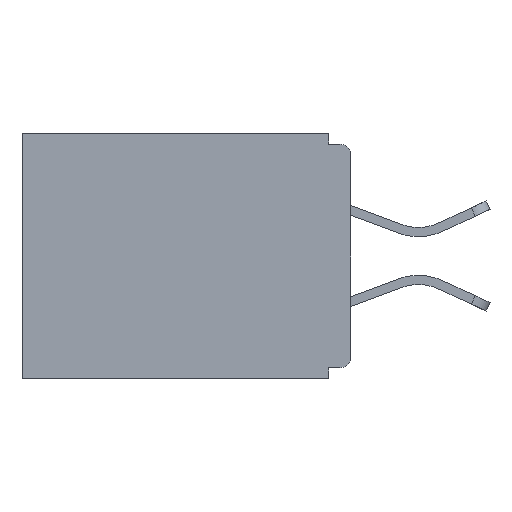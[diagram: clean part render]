
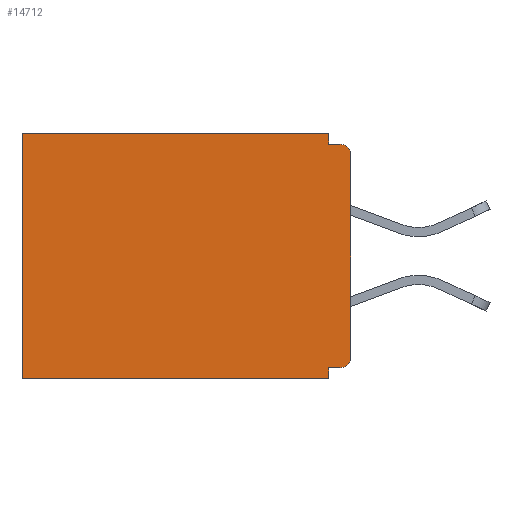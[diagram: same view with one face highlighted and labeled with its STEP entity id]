
A CAD part, left-side view. The second image highlights one B-rep face of the part: STEP entity #14712.
In plain terms, the highlighted planar face has unit normal (-1, 0, 0).
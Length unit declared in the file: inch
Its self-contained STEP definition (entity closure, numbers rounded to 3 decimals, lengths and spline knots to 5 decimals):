
#4 = CARTESIAN_POINT ( 'NONE',  ( 0.298, 0.031, -0.328 ) ) ;
#178 = LINE ( 'NONE', #515, #5808 ) ;
#179 = ORIENTED_EDGE ( 'NONE', *, *, #16428, .F. ) ;
#185 = CARTESIAN_POINT ( 'NONE',  ( 0.298, 0.031, -0.343 ) ) ;
#515 = CARTESIAN_POINT ( 'NONE',  ( 0.298, 0., -0.328 ) ) ;
#634 = CARTESIAN_POINT ( 'NONE',  ( 0.298, 0.46, 0. ) ) ;
#1150 = EDGE_CURVE ( 'NONE', #5513, #9753, #13021, .T. ) ;
#1374 = CARTESIAN_POINT ( 'NONE',  ( 0.298, 0.031, -0.343 ) ) ;
#1407 = EDGE_LOOP ( 'NONE', ( #13630, #1444, #7308, #13291, #6910, #11498, #1440, #179, #6808, #5266 ) ) ;
#1440 = ORIENTED_EDGE ( 'NONE', *, *, #1645, .F. ) ;
#1444 = ORIENTED_EDGE ( 'NONE', *, *, #9063, .F. ) ;
#1598 = VECTOR ( 'NONE', #7910, 39.37008 ) ;
#1629 = EDGE_CURVE ( 'NONE', #8692, #10953, #5450, .T. ) ;
#1645 = EDGE_CURVE ( 'NONE', #11223, #8692, #11439, .T. ) ;
#1943 = VECTOR ( 'NONE', #14411, 39.37008 ) ;
#2340 = VECTOR ( 'NONE', #9691, 39.37008 ) ;
#2417 = DIRECTION ( 'NONE',  ( 0., 0., -1. ) ) ;
#3238 = CARTESIAN_POINT ( 'NONE',  ( 0.298, 0., 0. ) ) ;
#3262 = EDGE_CURVE ( 'NONE', #7286, #14061, #7306, .T. ) ;
#3324 = VECTOR ( 'NONE', #3761, 39.37008 ) ;
#3612 = DIRECTION ( 'NONE',  ( -1., 0., 0. ) ) ;
#3679 = VECTOR ( 'NONE', #2417, 39.37008 ) ;
#3761 = DIRECTION ( 'NONE',  ( 0., 1., 0. ) ) ;
#4390 = LINE ( 'NONE', #634, #12402 ) ;
#4412 = PLANE ( 'NONE',  #11526 ) ;
#4455 = DIRECTION ( 'NONE',  ( 0., 1., 0. ) ) ;
#4909 = VERTEX_POINT ( 'NONE', #7822 ) ;
#5168 = CARTESIAN_POINT ( 'NONE',  ( 0.298, 0.015, -0.328 ) ) ;
#5172 = AXIS2_PLACEMENT_3D ( 'NONE', #9846, #3612, #14905 ) ;
#5266 = ORIENTED_EDGE ( 'NONE', *, *, #6485, .F. ) ;
#5450 = LINE ( 'NONE', #10848, #8223 ) ;
#5513 = VERTEX_POINT ( 'NONE', #13743 ) ;
#5716 = CARTESIAN_POINT ( 'NONE',  ( 0.298, 0., 0. ) ) ;
#5808 = VECTOR ( 'NONE', #8428, 39.37008 ) ;
#6282 = CARTESIAN_POINT ( 'NONE',  ( 0.298, 0., 0. ) ) ;
#6297 = CARTESIAN_POINT ( 'NONE',  ( 0.298, 0.031, -0.015 ) ) ;
#6485 = EDGE_CURVE ( 'NONE', #5513, #10709, #15809, .T. ) ;
#6808 = ORIENTED_EDGE ( 'NONE', *, *, #13981, .T. ) ;
#6819 = DIRECTION ( 'NONE',  ( 0., 0., -1. ) ) ;
#6910 = ORIENTED_EDGE ( 'NONE', *, *, #16467, .T. ) ;
#7286 = VERTEX_POINT ( 'NONE', #9744 ) ;
#7306 = LINE ( 'NONE', #1374, #3679 ) ;
#7308 = ORIENTED_EDGE ( 'NONE', *, *, #3262, .F. ) ;
#7575 = AXIS2_PLACEMENT_3D ( 'NONE', #11756, #14497, #6819 ) ;
#7822 = CARTESIAN_POINT ( 'NONE',  ( 0.298, 0.46, 0. ) ) ;
#7910 = DIRECTION ( 'NONE',  ( 0., 0., -1. ) ) ;
#7918 = CARTESIAN_POINT ( 'NONE',  ( 0.298, 0., -0.015 ) ) ;
#8223 = VECTOR ( 'NONE', #4455, 39.37008 ) ;
#8428 = DIRECTION ( 'NONE',  ( 0., 1., 0. ) ) ;
#8692 = VERTEX_POINT ( 'NONE', #13845 ) ;
#9063 = EDGE_CURVE ( 'NONE', #14061, #9753, #14378, .T. ) ;
#9455 = EDGE_CURVE ( 'NONE', #7286, #4909, #14975, .T. ) ;
#9556 = DIRECTION ( 'NONE',  ( 0., 0., -1. ) ) ;
#9691 = DIRECTION ( 'NONE',  ( 0., 0., -1. ) ) ;
#9744 = CARTESIAN_POINT ( 'NONE',  ( 0.298, 0.031, 0. ) ) ;
#9753 = VERTEX_POINT ( 'NONE', #12408 ) ;
#9846 = CARTESIAN_POINT ( 'NONE',  ( 0.298, 0.015, -0.313 ) ) ;
#9995 = CARTESIAN_POINT ( 'NONE',  ( 0.298, 0.46, -0.343 ) ) ;
#10709 = VERTEX_POINT ( 'NONE', #14428 ) ;
#10848 = CARTESIAN_POINT ( 'NONE',  ( 0.298, 0., -0.343 ) ) ;
#10953 = VERTEX_POINT ( 'NONE', #9995 ) ;
#11223 = VERTEX_POINT ( 'NONE', #4 ) ;
#11439 = LINE ( 'NONE', #185, #1598 ) ;
#11498 = ORIENTED_EDGE ( 'NONE', *, *, #1629, .F. ) ;
#11526 = AXIS2_PLACEMENT_3D ( 'NONE', #5716, #16015, #9556 ) ;
#11756 = CARTESIAN_POINT ( 'NONE',  ( 0.298, 0.015, -0.03 ) ) ;
#12219 = DIRECTION ( 'NONE',  ( 0., 0., -1. ) ) ;
#12402 = VECTOR ( 'NONE', #12219, 39.37008 ) ;
#12408 = CARTESIAN_POINT ( 'NONE',  ( 0.298, 0.015, -0.015 ) ) ;
#13021 = CIRCLE ( 'NONE', #7575, 0.015 ) ;
#13207 = CIRCLE ( 'NONE', #5172, 0.015 ) ;
#13291 = ORIENTED_EDGE ( 'NONE', *, *, #9455, .T. ) ;
#13630 = ORIENTED_EDGE ( 'NONE', *, *, #1150, .T. ) ;
#13743 = CARTESIAN_POINT ( 'NONE',  ( 0.298, 0., -0.03 ) ) ;
#13845 = CARTESIAN_POINT ( 'NONE',  ( 0.298, 0.031, -0.343 ) ) ;
#13981 = EDGE_CURVE ( 'NONE', #14967, #10709, #13207, .T. ) ;
#14061 = VERTEX_POINT ( 'NONE', #6297 ) ;
#14378 = LINE ( 'NONE', #7918, #1943 ) ;
#14411 = DIRECTION ( 'NONE',  ( 0., -1., 0. ) ) ;
#14428 = CARTESIAN_POINT ( 'NONE',  ( 0.298, 0., -0.313 ) ) ;
#14497 = DIRECTION ( 'NONE',  ( -1., 0., 0. ) ) ;
#14712 = ADVANCED_FACE ( 'NONE', ( #15023 ), #4412, .F. ) ;
#14905 = DIRECTION ( 'NONE',  ( 0., 0., -1. ) ) ;
#14967 = VERTEX_POINT ( 'NONE', #5168 ) ;
#14975 = LINE ( 'NONE', #6282, #3324 ) ;
#15023 = FACE_OUTER_BOUND ( 'NONE', #1407, .T. ) ;
#15809 = LINE ( 'NONE', #3238, #2340 ) ;
#16015 = DIRECTION ( 'NONE',  ( 1., 0., 0. ) ) ;
#16428 = EDGE_CURVE ( 'NONE', #14967, #11223, #178, .T. ) ;
#16467 = EDGE_CURVE ( 'NONE', #4909, #10953, #4390, .T. ) ;
